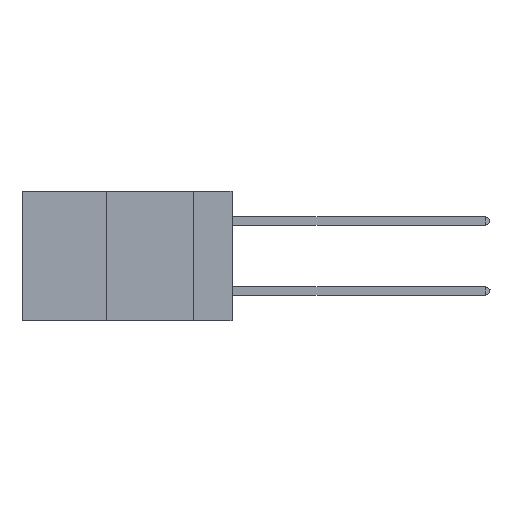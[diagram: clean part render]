
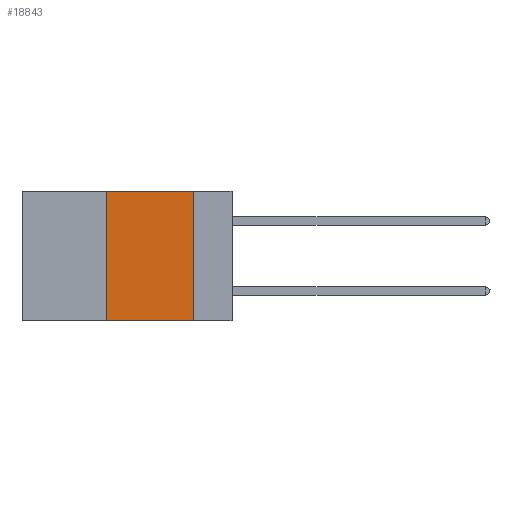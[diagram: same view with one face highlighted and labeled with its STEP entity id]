
A CAD part, left-side view. The second image highlights one B-rep face of the part: STEP entity #18843.
In plain terms, the highlighted planar face has unit normal (-1, 0, 0).
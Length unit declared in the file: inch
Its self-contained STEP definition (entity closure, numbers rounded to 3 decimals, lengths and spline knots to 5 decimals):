
#348 = CARTESIAN_POINT ( 'NONE',  ( 0., 0.36, 0. ) ) ;
#596 = ORIENTED_EDGE ( 'NONE', *, *, #11477, .F. ) ;
#1008 = LINE ( 'NONE', #29633, #12528 ) ;
#1240 = ORIENTED_EDGE ( 'NONE', *, *, #28983, .F. ) ;
#1588 = ORIENTED_EDGE ( 'NONE', *, *, #9318, .F. ) ;
#1911 = ORIENTED_EDGE ( 'NONE', *, *, #3002, .T. ) ;
#3002 = EDGE_CURVE ( 'NONE', #23001, #21927, #9481, .T. ) ;
#4048 = VERTEX_POINT ( 'NONE', #20862 ) ;
#4053 = DIRECTION ( 'NONE',  ( 0., 0., -1. ) ) ;
#4745 = AXIS2_PLACEMENT_3D ( 'NONE', #24676, #17860, #4053 ) ;
#5072 = CARTESIAN_POINT ( 'NONE',  ( 0., 0.36, -0.37 ) ) ;
#6060 = FACE_OUTER_BOUND ( 'NONE', #14164, .T. ) ;
#7412 = LINE ( 'NONE', #26933, #18212 ) ;
#9318 = EDGE_CURVE ( 'NONE', #23001, #25048, #22293, .T. ) ;
#9481 = LINE ( 'NONE', #9924, #21035 ) ;
#9924 = CARTESIAN_POINT ( 'NONE',  ( 0., 0.6, -0.37 ) ) ;
#11477 = EDGE_CURVE ( 'NONE', #4048, #21927, #7412, .T. ) ;
#12528 = VECTOR ( 'NONE', #13599, 39.37008 ) ;
#13179 = DIRECTION ( 'NONE',  ( 0., 0., -1. ) ) ;
#13599 = DIRECTION ( 'NONE',  ( 0., -1., 0. ) ) ;
#14164 = EDGE_LOOP ( 'NONE', ( #596, #1240, #1588, #1911 ) ) ;
#14332 = CARTESIAN_POINT ( 'NONE',  ( 0., 0.36, 0. ) ) ;
#15515 = PLANE ( 'NONE',  #4745 ) ;
#17860 = DIRECTION ( 'NONE',  ( 1., 0., 0. ) ) ;
#18212 = VECTOR ( 'NONE', #13179, 39.37008 ) ;
#18843 = ADVANCED_FACE ( 'NONE', ( #6060 ), #15515, .F. ) ;
#19246 = DIRECTION ( 'NONE',  ( 0., -1., 0. ) ) ;
#20862 = CARTESIAN_POINT ( 'NONE',  ( 0., 0.11, 0. ) ) ;
#21035 = VECTOR ( 'NONE', #19246, 39.37008 ) ;
#21927 = VERTEX_POINT ( 'NONE', #22033 ) ;
#22033 = CARTESIAN_POINT ( 'NONE',  ( 0., 0.11, -0.37 ) ) ;
#22293 = LINE ( 'NONE', #14332, #28309 ) ;
#23001 = VERTEX_POINT ( 'NONE', #5072 ) ;
#24676 = CARTESIAN_POINT ( 'NONE',  ( 0., 0.6, 0. ) ) ;
#25048 = VERTEX_POINT ( 'NONE', #348 ) ;
#25792 = DIRECTION ( 'NONE',  ( 0., 0., 1. ) ) ;
#26933 = CARTESIAN_POINT ( 'NONE',  ( 0., 0.11, 0. ) ) ;
#28309 = VECTOR ( 'NONE', #25792, 39.37008 ) ;
#28983 = EDGE_CURVE ( 'NONE', #25048, #4048, #1008, .T. ) ;
#29633 = CARTESIAN_POINT ( 'NONE',  ( 0., 0.6, 0. ) ) ;
